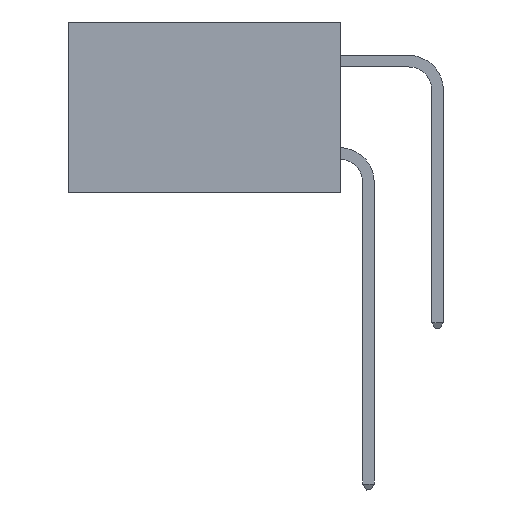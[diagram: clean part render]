
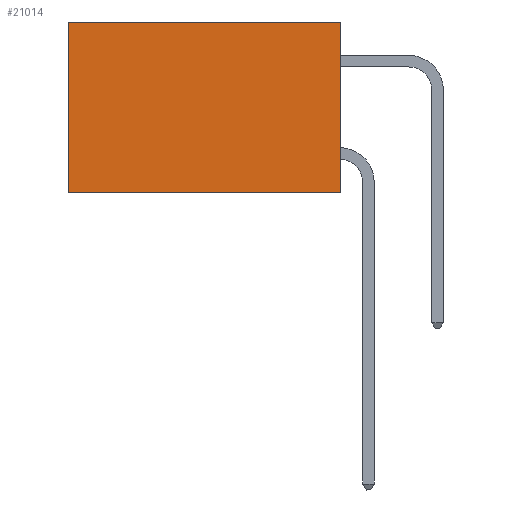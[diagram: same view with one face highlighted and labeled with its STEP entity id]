
A CAD part, left-side view. The second image highlights one B-rep face of the part: STEP entity #21014.
In plain terms, the highlighted planar face has unit normal (-1, 0, 0).
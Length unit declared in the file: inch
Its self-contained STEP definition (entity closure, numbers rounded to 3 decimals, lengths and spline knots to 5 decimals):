
#267 = EDGE_CURVE ( 'NONE', #5017, #14264, #9843, .T. ) ;
#942 = DIRECTION ( 'NONE',  ( 0., 0., -1. ) ) ;
#1058 = CARTESIAN_POINT ( 'NONE',  ( 0.277, 0., -0.37 ) ) ;
#1227 = VECTOR ( 'NONE', #17407, 39.37008 ) ;
#3391 = VERTEX_POINT ( 'NONE', #1058 ) ;
#3454 = PLANE ( 'NONE',  #13441 ) ;
#3959 = VECTOR ( 'NONE', #13071, 39.37008 ) ;
#4070 = VERTEX_POINT ( 'NONE', #4592 ) ;
#4467 = DIRECTION ( 'NONE',  ( 0., 0., -1. ) ) ;
#4592 = CARTESIAN_POINT ( 'NONE',  ( 0.277, 0., 0. ) ) ;
#5017 = VERTEX_POINT ( 'NONE', #20135 ) ;
#8782 = DIRECTION ( 'NONE',  ( 1., 0., 0. ) ) ;
#9694 = CARTESIAN_POINT ( 'NONE',  ( 0.277, 0., -0.37 ) ) ;
#9843 = LINE ( 'NONE', #20841, #14002 ) ;
#10589 = LINE ( 'NONE', #15652, #1227 ) ;
#12838 = ORIENTED_EDGE ( 'NONE', *, *, #267, .T. ) ;
#13071 = DIRECTION ( 'NONE',  ( 0., 1., 0. ) ) ;
#13441 = AXIS2_PLACEMENT_3D ( 'NONE', #19334, #8782, #21123 ) ;
#13604 = FACE_OUTER_BOUND ( 'NONE', #17367, .T. ) ;
#13637 = ORIENTED_EDGE ( 'NONE', *, *, #16944, .T. ) ;
#13926 = CARTESIAN_POINT ( 'NONE',  ( 0.277, 0.59, -0.37 ) ) ;
#14002 = VECTOR ( 'NONE', #4467, 39.37008 ) ;
#14264 = VERTEX_POINT ( 'NONE', #13926 ) ;
#15405 = EDGE_CURVE ( 'NONE', #4070, #3391, #16728, .T. ) ;
#15652 = CARTESIAN_POINT ( 'NONE',  ( 0.277, 0., -0.37 ) ) ;
#16513 = CARTESIAN_POINT ( 'NONE',  ( 0.277, 0., 0. ) ) ;
#16728 = LINE ( 'NONE', #9694, #20891 ) ;
#16944 = EDGE_CURVE ( 'NONE', #4070, #5017, #18051, .T. ) ;
#17367 = EDGE_LOOP ( 'NONE', ( #12838, #21512, #20783, #13637 ) ) ;
#17407 = DIRECTION ( 'NONE',  ( 0., 1., 0. ) ) ;
#18051 = LINE ( 'NONE', #16513, #3959 ) ;
#19334 = CARTESIAN_POINT ( 'NONE',  ( 0.277, 0., -0.37 ) ) ;
#20135 = CARTESIAN_POINT ( 'NONE',  ( 0.277, 0.59, 0. ) ) ;
#20783 = ORIENTED_EDGE ( 'NONE', *, *, #15405, .F. ) ;
#20841 = CARTESIAN_POINT ( 'NONE',  ( 0.277, 0.59, -0.37 ) ) ;
#20891 = VECTOR ( 'NONE', #942, 39.37008 ) ;
#20947 = EDGE_CURVE ( 'NONE', #3391, #14264, #10589, .T. ) ;
#21014 = ADVANCED_FACE ( 'NONE', ( #13604 ), #3454, .F. ) ;
#21123 = DIRECTION ( 'NONE',  ( 0., 0., -1. ) ) ;
#21512 = ORIENTED_EDGE ( 'NONE', *, *, #20947, .F. ) ;
